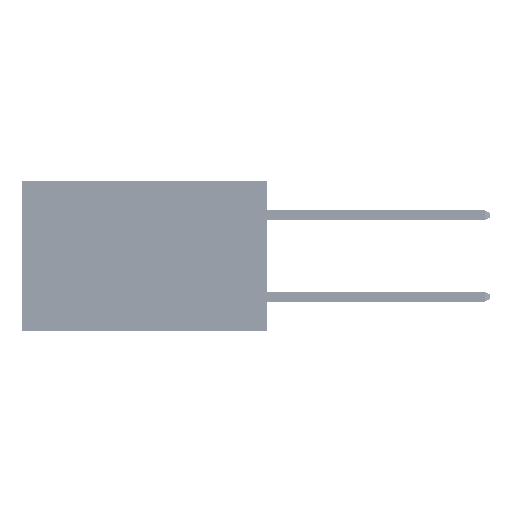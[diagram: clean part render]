
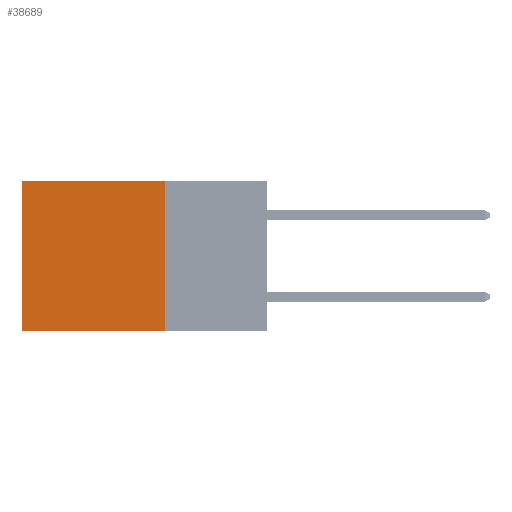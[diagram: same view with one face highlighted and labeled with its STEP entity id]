
A CAD part, left-side view. The second image highlights one B-rep face of the part: STEP entity #38689.
In plain terms, the highlighted planar face has unit normal (-1, 0, 0).
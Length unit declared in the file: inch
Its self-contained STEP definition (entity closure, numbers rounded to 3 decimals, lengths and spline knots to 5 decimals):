
#1543 = LINE ( 'NONE', #50234, #18663 ) ;
#2938 = CARTESIAN_POINT ( 'NONE',  ( 0.2875, 0.6, 0. ) ) ;
#4029 = VERTEX_POINT ( 'NONE', #35359 ) ;
#4532 = DIRECTION ( 'NONE',  ( 0., 1., 0. ) ) ;
#5829 = AXIS2_PLACEMENT_3D ( 'NONE', #17979, #37414, #17625 ) ;
#11837 = LINE ( 'NONE', #45079, #37157 ) ;
#12977 = ORIENTED_EDGE ( 'NONE', *, *, #29842, .F. ) ;
#13352 = VERTEX_POINT ( 'NONE', #19944 ) ;
#16098 = EDGE_LOOP ( 'NONE', ( #18849, #12977, #42368, #35212 ) ) ;
#17625 = DIRECTION ( 'NONE',  ( 0., 0., -1. ) ) ;
#17979 = CARTESIAN_POINT ( 'NONE',  ( 0.2875, 0.25, 0. ) ) ;
#18663 = VECTOR ( 'NONE', #41927, 39.37008 ) ;
#18849 = ORIENTED_EDGE ( 'NONE', *, *, #25203, .T. ) ;
#19944 = CARTESIAN_POINT ( 'NONE',  ( 0.2875, 0.6, 0. ) ) ;
#21681 = DIRECTION ( 'NONE',  ( 0., 0., -1. ) ) ;
#22440 = LINE ( 'NONE', #2938, #52155 ) ;
#25203 = EDGE_CURVE ( 'NONE', #13352, #44999, #22440, .T. ) ;
#25559 = CARTESIAN_POINT ( 'NONE',  ( 0.2875, 0.25, 0. ) ) ;
#26724 = CARTESIAN_POINT ( 'NONE',  ( 0.2875, 0.6, -0.37 ) ) ;
#29842 = EDGE_CURVE ( 'NONE', #4029, #44999, #11837, .T. ) ;
#34309 = VECTOR ( 'NONE', #21681, 39.37008 ) ;
#35212 = ORIENTED_EDGE ( 'NONE', *, *, #37508, .T. ) ;
#35359 = CARTESIAN_POINT ( 'NONE',  ( 0.2875, 0.25, -0.37 ) ) ;
#37157 = VECTOR ( 'NONE', #4532, 39.37008 ) ;
#37414 = DIRECTION ( 'NONE',  ( 1., 0., 0. ) ) ;
#37508 = EDGE_CURVE ( 'NONE', #50735, #13352, #1543, .T. ) ;
#38689 = ADVANCED_FACE ( 'NONE', ( #50777 ), #45558, .F. ) ;
#41927 = DIRECTION ( 'NONE',  ( 0., 1., 0. ) ) ;
#42368 = ORIENTED_EDGE ( 'NONE', *, *, #50581, .F. ) ;
#43189 = LINE ( 'NONE', #49942, #34309 ) ;
#44999 = VERTEX_POINT ( 'NONE', #26724 ) ;
#45079 = CARTESIAN_POINT ( 'NONE',  ( 0.2875, 0.25, -0.37 ) ) ;
#45558 = PLANE ( 'NONE',  #5829 ) ;
#49942 = CARTESIAN_POINT ( 'NONE',  ( 0.2875, 0.25, 0. ) ) ;
#50234 = CARTESIAN_POINT ( 'NONE',  ( 0.2875, 0.25, 0. ) ) ;
#50581 = EDGE_CURVE ( 'NONE', #50735, #4029, #43189, .T. ) ;
#50735 = VERTEX_POINT ( 'NONE', #25559 ) ;
#50777 = FACE_OUTER_BOUND ( 'NONE', #16098, .T. ) ;
#51597 = DIRECTION ( 'NONE',  ( 0., 0., -1. ) ) ;
#52155 = VECTOR ( 'NONE', #51597, 39.37008 ) ;
